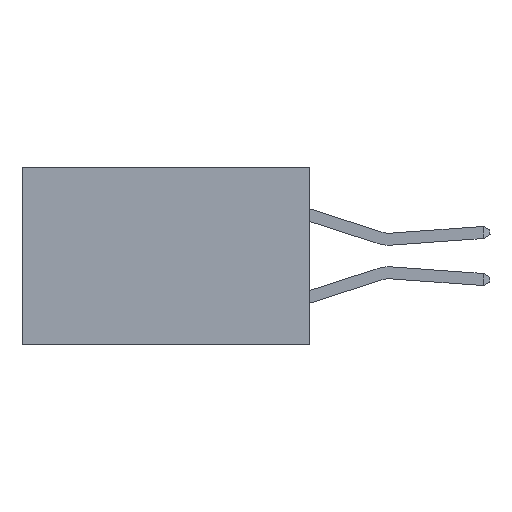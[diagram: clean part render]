
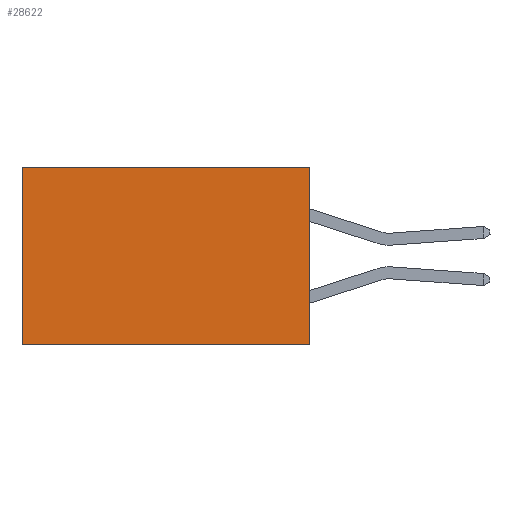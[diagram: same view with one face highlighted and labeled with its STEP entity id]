
A CAD part, left-side view. The second image highlights one B-rep face of the part: STEP entity #28622.
In plain terms, the highlighted planar face has unit normal (-1, 0, 0).
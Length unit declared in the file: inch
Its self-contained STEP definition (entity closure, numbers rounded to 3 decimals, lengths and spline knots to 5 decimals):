
#759 = VECTOR ( 'NONE', #15504, 39.37008 ) ;
#1066 = EDGE_CURVE ( 'NONE', #25448, #30789, #29986, .T. ) ;
#1403 = FACE_OUTER_BOUND ( 'NONE', #3183, .T. ) ;
#1703 = CARTESIAN_POINT ( 'NONE',  ( 0.298, 0., -0.37 ) ) ;
#1808 = ORIENTED_EDGE ( 'NONE', *, *, #9932, .F. ) ;
#2998 = VECTOR ( 'NONE', #19783, 39.37008 ) ;
#3183 = EDGE_LOOP ( 'NONE', ( #9388, #19230, #1808, #16912 ) ) ;
#4380 = CARTESIAN_POINT ( 'NONE',  ( 0.298, 0., 0. ) ) ;
#5926 = LINE ( 'NONE', #15179, #24672 ) ;
#6507 = CARTESIAN_POINT ( 'NONE',  ( 0.298, 0., 0. ) ) ;
#6817 = PLANE ( 'NONE',  #24107 ) ;
#8605 = VERTEX_POINT ( 'NONE', #6507 ) ;
#9388 = ORIENTED_EDGE ( 'NONE', *, *, #16523, .T. ) ;
#9932 = EDGE_CURVE ( 'NONE', #8605, #25448, #5926, .T. ) ;
#10418 = VECTOR ( 'NONE', #31189, 39.37008 ) ;
#10612 = CARTESIAN_POINT ( 'NONE',  ( 0.298, 0.6, 0. ) ) ;
#10971 = LINE ( 'NONE', #26381, #2998 ) ;
#12923 = DIRECTION ( 'NONE',  ( 0., 0., -1. ) ) ;
#14084 = DIRECTION ( 'NONE',  ( 1., 0., 0. ) ) ;
#14983 = VERTEX_POINT ( 'NONE', #10612 ) ;
#15179 = CARTESIAN_POINT ( 'NONE',  ( 0.298, 0., 0. ) ) ;
#15504 = DIRECTION ( 'NONE',  ( 0., 0., -1. ) ) ;
#16523 = EDGE_CURVE ( 'NONE', #14983, #30789, #19139, .T. ) ;
#16912 = ORIENTED_EDGE ( 'NONE', *, *, #28677, .T. ) ;
#19139 = LINE ( 'NONE', #30222, #759 ) ;
#19230 = ORIENTED_EDGE ( 'NONE', *, *, #1066, .F. ) ;
#19783 = DIRECTION ( 'NONE',  ( 0., 1., 0. ) ) ;
#24053 = DIRECTION ( 'NONE',  ( 0., 0., -1. ) ) ;
#24107 = AXIS2_PLACEMENT_3D ( 'NONE', #4380, #14084, #24053 ) ;
#24672 = VECTOR ( 'NONE', #12923, 39.37008 ) ;
#25448 = VERTEX_POINT ( 'NONE', #28266 ) ;
#26381 = CARTESIAN_POINT ( 'NONE',  ( 0.298, 0., 0. ) ) ;
#28266 = CARTESIAN_POINT ( 'NONE',  ( 0.298, 0., -0.37 ) ) ;
#28622 = ADVANCED_FACE ( 'NONE', ( #1403 ), #6817, .F. ) ;
#28677 = EDGE_CURVE ( 'NONE', #8605, #14983, #10971, .T. ) ;
#29094 = CARTESIAN_POINT ( 'NONE',  ( 0.298, 0.6, -0.37 ) ) ;
#29986 = LINE ( 'NONE', #1703, #10418 ) ;
#30222 = CARTESIAN_POINT ( 'NONE',  ( 0.298, 0.6, 0. ) ) ;
#30789 = VERTEX_POINT ( 'NONE', #29094 ) ;
#31189 = DIRECTION ( 'NONE',  ( 0., 1., 0. ) ) ;
